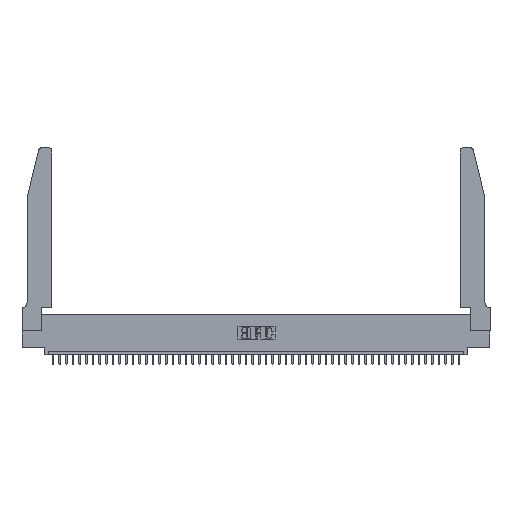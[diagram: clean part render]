
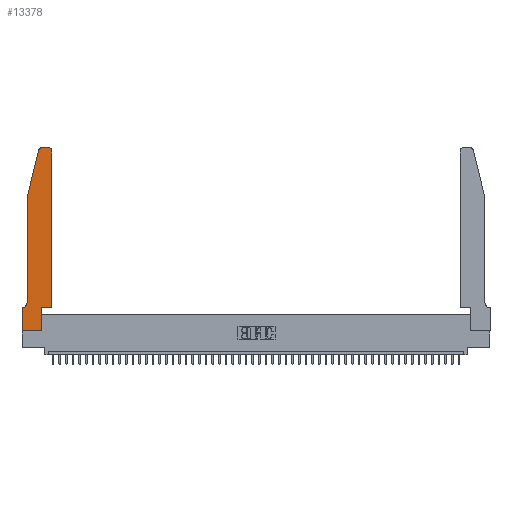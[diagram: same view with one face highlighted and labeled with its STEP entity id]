
A CAD part, top view. The second image highlights one B-rep face of the part: STEP entity #13378.
In plain terms, the highlighted planar face has unit normal (0, 0, 1).
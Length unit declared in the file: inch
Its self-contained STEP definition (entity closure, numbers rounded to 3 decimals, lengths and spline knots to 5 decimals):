
#511 = ORIENTED_EDGE ( 'NONE', *, *, #9214, .T. ) ;
#1737 = CARTESIAN_POINT ( 'NONE',  ( 0.0055, 0.35, 0.37 ) ) ;
#1824 = LINE ( 'NONE', #43667, #38490 ) ;
#2414 = VERTEX_POINT ( 'NONE', #45322 ) ;
#2512 = ORIENTED_EDGE ( 'NONE', *, *, #17824, .T. ) ;
#3705 = EDGE_CURVE ( 'NONE', #45961, #2414, #15425, .T. ) ;
#5474 = DIRECTION ( 'NONE',  ( 1., 0., 0. ) ) ;
#5875 = ORIENTED_EDGE ( 'NONE', *, *, #47936, .T. ) ;
#6059 = DIRECTION ( 'NONE',  ( 1., 0., 0. ) ) ;
#6432 = LINE ( 'NONE', #30612, #37758 ) ;
#6656 = CIRCLE ( 'NONE', #16251, 0.03 ) ;
#6681 = DIRECTION ( 'NONE',  ( -0.239, -0.971, 0. ) ) ;
#7631 = VECTOR ( 'NONE', #21151, 39.37008 ) ;
#8011 = DIRECTION ( 'NONE',  ( 1., 0., 0. ) ) ;
#8029 = ORIENTED_EDGE ( 'NONE', *, *, #47121, .T. ) ;
#8345 = AXIS2_PLACEMENT_3D ( 'NONE', #30586, #15597, #8011 ) ;
#9214 = EDGE_CURVE ( 'NONE', #33010, #45961, #24548, .T. ) ;
#9264 = CIRCLE ( 'NONE', #20602, 0.07 ) ;
#9656 = DIRECTION ( 'NONE',  ( 0., 0., -1. ) ) ;
#9810 = ORIENTED_EDGE ( 'NONE', *, *, #26696, .T. ) ;
#11792 = LINE ( 'NONE', #12742, #30665 ) ;
#12023 = CARTESIAN_POINT ( 'NONE',  ( 0.4505, 0.35, 0.37 ) ) ;
#12742 = CARTESIAN_POINT ( 'NONE',  ( 0.2605, 2.75, 0.37 ) ) ;
#13378 = ADVANCED_FACE ( 'NONE', ( #26743 ), #25933, .T. ) ;
#15191 = VERTEX_POINT ( 'NONE', #24810 ) ;
#15425 = LINE ( 'NONE', #40603, #48548 ) ;
#15462 = LINE ( 'NONE', #45563, #45047 ) ;
#15516 = EDGE_CURVE ( 'NONE', #15191, #19375, #11792, .T. ) ;
#15597 = DIRECTION ( 'NONE',  ( 0., 0., 1. ) ) ;
#16251 = AXIS2_PLACEMENT_3D ( 'NONE', #25701, #26033, #48520 ) ;
#16344 = VECTOR ( 'NONE', #25138, 39.37008 ) ;
#17170 = CARTESIAN_POINT ( 'NONE',  ( 0.0755, 0.42, 0.37 ) ) ;
#17654 = LINE ( 'NONE', #46930, #7631 ) ;
#17824 = EDGE_CURVE ( 'NONE', #31901, #33010, #37073, .T. ) ;
#17907 = CARTESIAN_POINT ( 'NONE',  ( 0.2865, 0., 0.37 ) ) ;
#19375 = VERTEX_POINT ( 'NONE', #25746 ) ;
#19609 = DIRECTION ( 'NONE',  ( 1., 0., 0. ) ) ;
#19823 = EDGE_CURVE ( 'NONE', #45669, #22200, #1824, .T. ) ;
#20146 = DIRECTION ( 'NONE',  ( -1., 0., 0. ) ) ;
#20293 = ORIENTED_EDGE ( 'NONE', *, *, #39944, .T. ) ;
#20412 = CARTESIAN_POINT ( 'NONE',  ( 0.4505, 0.35, 0.37 ) ) ;
#20430 = ORIENTED_EDGE ( 'NONE', *, *, #15516, .T. ) ;
#20602 = AXIS2_PLACEMENT_3D ( 'NONE', #32080, #9656, #46965 ) ;
#21151 = DIRECTION ( 'NONE',  ( 0., -1., 0. ) ) ;
#21433 = DIRECTION ( 'NONE',  ( 0., -1., 0. ) ) ;
#22200 = VERTEX_POINT ( 'NONE', #45317 ) ;
#23435 = EDGE_CURVE ( 'NONE', #41375, #46472, #9264, .T. ) ;
#23547 = DIRECTION ( 'NONE',  ( -1., 0., 0. ) ) ;
#24070 = ORIENTED_EDGE ( 'NONE', *, *, #23435, .T. ) ;
#24548 = LINE ( 'NONE', #20412, #48776 ) ;
#24810 = CARTESIAN_POINT ( 'NONE',  ( 0.4205, 2.75, 0.37 ) ) ;
#25138 = DIRECTION ( 'NONE',  ( 0., 1., 0. ) ) ;
#25408 = EDGE_LOOP ( 'NONE', ( #20430, #9810, #47829, #5875, #24070, #20293, #8029, #32737, #2512, #511, #45494, #37842 ) ) ;
#25701 = CARTESIAN_POINT ( 'NONE',  ( 0.284, 2.72, 0.37 ) ) ;
#25746 = CARTESIAN_POINT ( 'NONE',  ( 0.284, 2.75, 0.37 ) ) ;
#25933 = PLANE ( 'NONE',  #26559 ) ;
#25978 = CIRCLE ( 'NONE', #8345, 0.03 ) ;
#26033 = DIRECTION ( 'NONE',  ( 0., 0., 1. ) ) ;
#26493 = EDGE_CURVE ( 'NONE', #41513, #31901, #15462, .T. ) ;
#26559 = AXIS2_PLACEMENT_3D ( 'NONE', #42804, #46558, #5474 ) ;
#26696 = EDGE_CURVE ( 'NONE', #19375, #45669, #6656, .T. ) ;
#26743 = FACE_OUTER_BOUND ( 'NONE', #25408, .T. ) ;
#29038 = CARTESIAN_POINT ( 'NONE',  ( 0.2865, 0.35, 0.37 ) ) ;
#30586 = CARTESIAN_POINT ( 'NONE',  ( 0.4205, 2.72, 0.37 ) ) ;
#30612 = CARTESIAN_POINT ( 'NONE',  ( 0.0755, 0.35, 0.37 ) ) ;
#30665 = VECTOR ( 'NONE', #20146, 39.37008 ) ;
#31901 = VERTEX_POINT ( 'NONE', #17907 ) ;
#32080 = CARTESIAN_POINT ( 'NONE',  ( 0.0055, 0.42, 0.37 ) ) ;
#32737 = ORIENTED_EDGE ( 'NONE', *, *, #26493, .T. ) ;
#32790 = CARTESIAN_POINT ( 'NONE',  ( 0.0755, 2., 0.37 ) ) ;
#33010 = VERTEX_POINT ( 'NONE', #44008 ) ;
#36864 = CARTESIAN_POINT ( 'NONE',  ( 0., 0.35, 0.37 ) ) ;
#37073 = LINE ( 'NONE', #29038, #16344 ) ;
#37131 = VECTOR ( 'NONE', #21433, 39.37008 ) ;
#37758 = VECTOR ( 'NONE', #23547, 39.37008 ) ;
#37842 = ORIENTED_EDGE ( 'NONE', *, *, #48169, .T. ) ;
#38490 = VECTOR ( 'NONE', #6681, 39.37008 ) ;
#38968 = LINE ( 'NONE', #32790, #37131 ) ;
#39625 = CARTESIAN_POINT ( 'NONE',  ( 0.25487, 2.72718, 0.37 ) ) ;
#39944 = EDGE_CURVE ( 'NONE', #46472, #41420, #6432, .T. ) ;
#40603 = CARTESIAN_POINT ( 'NONE',  ( 0.4505, 0.35, 0.37 ) ) ;
#41375 = VERTEX_POINT ( 'NONE', #17170 ) ;
#41420 = VERTEX_POINT ( 'NONE', #36864 ) ;
#41513 = VERTEX_POINT ( 'NONE', #47744 ) ;
#42804 = CARTESIAN_POINT ( 'NONE',  ( 0., 0.35, 0.37 ) ) ;
#43667 = CARTESIAN_POINT ( 'NONE',  ( 0.0755, 2., 0.37 ) ) ;
#44008 = CARTESIAN_POINT ( 'NONE',  ( 0.2865, 0.35, 0.37 ) ) ;
#45047 = VECTOR ( 'NONE', #19609, 39.37008 ) ;
#45317 = CARTESIAN_POINT ( 'NONE',  ( 0.0755, 2., 0.37 ) ) ;
#45322 = CARTESIAN_POINT ( 'NONE',  ( 0.4505, 2.72, 0.37 ) ) ;
#45494 = ORIENTED_EDGE ( 'NONE', *, *, #3705, .T. ) ;
#45563 = CARTESIAN_POINT ( 'NONE',  ( 0., 0., 0.37 ) ) ;
#45669 = VERTEX_POINT ( 'NONE', #39625 ) ;
#45961 = VERTEX_POINT ( 'NONE', #12023 ) ;
#46472 = VERTEX_POINT ( 'NONE', #1737 ) ;
#46558 = DIRECTION ( 'NONE',  ( 0., 0., 1. ) ) ;
#46930 = CARTESIAN_POINT ( 'NONE',  ( 0., 0., 0.37 ) ) ;
#46965 = DIRECTION ( 'NONE',  ( -1., 0., 0. ) ) ;
#47121 = EDGE_CURVE ( 'NONE', #41420, #41513, #17654, .T. ) ;
#47744 = CARTESIAN_POINT ( 'NONE',  ( 0., 0., 0.37 ) ) ;
#47829 = ORIENTED_EDGE ( 'NONE', *, *, #19823, .T. ) ;
#47936 = EDGE_CURVE ( 'NONE', #22200, #41375, #38968, .T. ) ;
#48169 = EDGE_CURVE ( 'NONE', #2414, #15191, #25978, .T. ) ;
#48520 = DIRECTION ( 'NONE',  ( 1., 0., 0. ) ) ;
#48548 = VECTOR ( 'NONE', #48799, 39.37008 ) ;
#48776 = VECTOR ( 'NONE', #6059, 39.37008 ) ;
#48799 = DIRECTION ( 'NONE',  ( 0., 1., 0. ) ) ;
